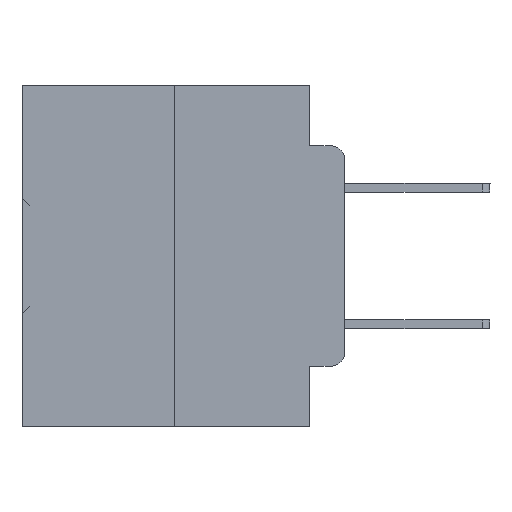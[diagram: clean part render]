
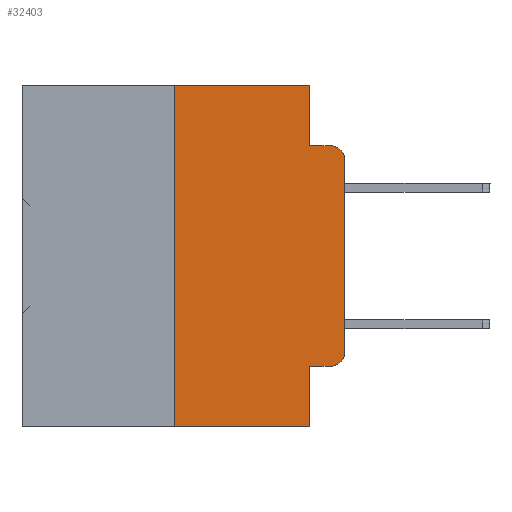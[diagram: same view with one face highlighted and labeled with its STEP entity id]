
A CAD part, left-side view. The second image highlights one B-rep face of the part: STEP entity #32403.
In plain terms, the highlighted planar face has unit normal (-1, 0, 0).
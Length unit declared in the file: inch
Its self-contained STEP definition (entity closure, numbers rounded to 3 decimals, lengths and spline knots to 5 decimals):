
#137 = PLANE ( 'NONE',  #22142 ) ;
#1534 = DIRECTION ( 'NONE',  ( 0., 0., 1. ) ) ;
#2020 = VECTOR ( 'NONE', #23748, 39.37008 ) ;
#2094 = CARTESIAN_POINT ( 'NONE',  ( 0., 0.051, -0.0885 ) ) ;
#2746 = ORIENTED_EDGE ( 'NONE', *, *, #9383, .T. ) ;
#2967 = VECTOR ( 'NONE', #6515, 39.37008 ) ;
#2983 = DIRECTION ( 'NONE',  ( 0., 0., -1. ) ) ;
#3300 = CIRCLE ( 'NONE', #10174, 0.02 ) ;
#3386 = CARTESIAN_POINT ( 'NONE',  ( 0., 0.051, 0. ) ) ;
#4355 = VERTEX_POINT ( 'NONE', #10969 ) ;
#4453 = CARTESIAN_POINT ( 'NONE',  ( 0., 0.02, -0.4115 ) ) ;
#4884 = VECTOR ( 'NONE', #2983, 39.37008 ) ;
#5462 = CARTESIAN_POINT ( 'NONE',  ( 0., 0.473, 0. ) ) ;
#5579 = DIRECTION ( 'NONE',  ( 0., -1., 0. ) ) ;
#6475 = VECTOR ( 'NONE', #10000, 39.37008 ) ;
#6515 = DIRECTION ( 'NONE',  ( 0., 0., -1. ) ) ;
#6992 = CARTESIAN_POINT ( 'NONE',  ( 0., 0.25, -0.5 ) ) ;
#7221 = EDGE_CURVE ( 'NONE', #24840, #11755, #3300, .T. ) ;
#7809 = LINE ( 'NONE', #16833, #32622 ) ;
#8378 = EDGE_CURVE ( 'NONE', #14174, #4355, #33177, .T. ) ;
#8612 = VERTEX_POINT ( 'NONE', #2094 ) ;
#8618 = ORIENTED_EDGE ( 'NONE', *, *, #7221, .T. ) ;
#9383 = EDGE_CURVE ( 'NONE', #11755, #16154, #34414, .T. ) ;
#9422 = CARTESIAN_POINT ( 'NONE',  ( 0., 0.051, 0. ) ) ;
#10000 = DIRECTION ( 'NONE',  ( 0., 0., 1. ) ) ;
#10174 = AXIS2_PLACEMENT_3D ( 'NONE', #35438, #23811, #29338 ) ;
#10324 = DIRECTION ( 'NONE',  ( 0., 0., -1. ) ) ;
#10969 = CARTESIAN_POINT ( 'NONE',  ( 0., 0.051, -0.5 ) ) ;
#11247 = ORIENTED_EDGE ( 'NONE', *, *, #12398, .F. ) ;
#11578 = DIRECTION ( 'NONE',  ( 0., -1., 0. ) ) ;
#11660 = CARTESIAN_POINT ( 'NONE',  ( 0., 0., -0.3915 ) ) ;
#11755 = VERTEX_POINT ( 'NONE', #11660 ) ;
#11783 = CARTESIAN_POINT ( 'NONE',  ( 0., 0.051, -0.0885 ) ) ;
#11917 = ORIENTED_EDGE ( 'NONE', *, *, #14824, .F. ) ;
#12398 = EDGE_CURVE ( 'NONE', #22626, #8612, #29917, .T. ) ;
#13065 = CARTESIAN_POINT ( 'NONE',  ( 0., 0.25, 0. ) ) ;
#13457 = CARTESIAN_POINT ( 'NONE',  ( 0., 0.051, -0.4115 ) ) ;
#14174 = VERTEX_POINT ( 'NONE', #6992 ) ;
#14824 = EDGE_CURVE ( 'NONE', #26205, #22626, #32669, .T. ) ;
#15072 = EDGE_CURVE ( 'NONE', #34968, #4355, #34246, .T. ) ;
#15093 = LINE ( 'NONE', #11783, #15556 ) ;
#15556 = VECTOR ( 'NONE', #11578, 39.37008 ) ;
#16154 = VERTEX_POINT ( 'NONE', #24230 ) ;
#16574 = EDGE_CURVE ( 'NONE', #8612, #32099, #15093, .T. ) ;
#16833 = CARTESIAN_POINT ( 'NONE',  ( 0., 0.25, 0. ) ) ;
#17112 = ORIENTED_EDGE ( 'NONE', *, *, #15072, .F. ) ;
#19751 = DIRECTION ( 'NONE',  ( -1., 0., 0. ) ) ;
#20144 = ORIENTED_EDGE ( 'NONE', *, *, #32571, .T. ) ;
#20518 = VECTOR ( 'NONE', #36239, 39.37008 ) ;
#22142 = AXIS2_PLACEMENT_3D ( 'NONE', #5462, #29257, #32967 ) ;
#22626 = VERTEX_POINT ( 'NONE', #28532 ) ;
#22902 = CARTESIAN_POINT ( 'NONE',  ( 0., 0.02, -0.1085 ) ) ;
#23243 = ORIENTED_EDGE ( 'NONE', *, *, #36819, .T. ) ;
#23748 = DIRECTION ( 'NONE',  ( 0., -1., 0. ) ) ;
#23811 = DIRECTION ( 'NONE',  ( -1., 0., 0. ) ) ;
#23840 = LINE ( 'NONE', #32511, #27478 ) ;
#24230 = CARTESIAN_POINT ( 'NONE',  ( 0., 0., -0.1085 ) ) ;
#24840 = VERTEX_POINT ( 'NONE', #4453 ) ;
#26205 = VERTEX_POINT ( 'NONE', #13065 ) ;
#27478 = VECTOR ( 'NONE', #5579, 39.37008 ) ;
#27689 = EDGE_CURVE ( 'NONE', #14174, #26205, #7809, .T. ) ;
#28532 = CARTESIAN_POINT ( 'NONE',  ( 0., 0.051, 0. ) ) ;
#28800 = ORIENTED_EDGE ( 'NONE', *, *, #27689, .F. ) ;
#29024 = ORIENTED_EDGE ( 'NONE', *, *, #16574, .F. ) ;
#29257 = DIRECTION ( 'NONE',  ( 1., 0., 0. ) ) ;
#29338 = DIRECTION ( 'NONE',  ( 0., 0., -1. ) ) ;
#29528 = CARTESIAN_POINT ( 'NONE',  ( 0., 0.473, 0. ) ) ;
#29917 = LINE ( 'NONE', #9422, #4884 ) ;
#30045 = CARTESIAN_POINT ( 'NONE',  ( 0., 0.473, -0.5 ) ) ;
#30321 = CIRCLE ( 'NONE', #35357, 0.02 ) ;
#31240 = CARTESIAN_POINT ( 'NONE',  ( 0., 0.02, -0.0885 ) ) ;
#31264 = CARTESIAN_POINT ( 'NONE',  ( 0., 0., 0. ) ) ;
#32099 = VERTEX_POINT ( 'NONE', #31240 ) ;
#32403 = ADVANCED_FACE ( 'NONE', ( #38313 ), #137, .F. ) ;
#32511 = CARTESIAN_POINT ( 'NONE',  ( 0., 0.051, -0.4115 ) ) ;
#32571 = EDGE_CURVE ( 'NONE', #16154, #32099, #30321, .T. ) ;
#32622 = VECTOR ( 'NONE', #1534, 39.37008 ) ;
#32669 = LINE ( 'NONE', #29528, #20518 ) ;
#32967 = DIRECTION ( 'NONE',  ( 0., 0., -1. ) ) ;
#33177 = LINE ( 'NONE', #30045, #2020 ) ;
#34246 = LINE ( 'NONE', #3386, #2967 ) ;
#34414 = LINE ( 'NONE', #31264, #6475 ) ;
#34920 = ORIENTED_EDGE ( 'NONE', *, *, #8378, .T. ) ;
#34968 = VERTEX_POINT ( 'NONE', #13457 ) ;
#35086 = EDGE_LOOP ( 'NONE', ( #2746, #20144, #29024, #11247, #11917, #28800, #34920, #17112, #23243, #8618 ) ) ;
#35357 = AXIS2_PLACEMENT_3D ( 'NONE', #22902, #19751, #10324 ) ;
#35438 = CARTESIAN_POINT ( 'NONE',  ( 0., 0.02, -0.3915 ) ) ;
#36239 = DIRECTION ( 'NONE',  ( 0., -1., 0. ) ) ;
#36819 = EDGE_CURVE ( 'NONE', #34968, #24840, #23840, .T. ) ;
#38313 = FACE_OUTER_BOUND ( 'NONE', #35086, .T. ) ;
